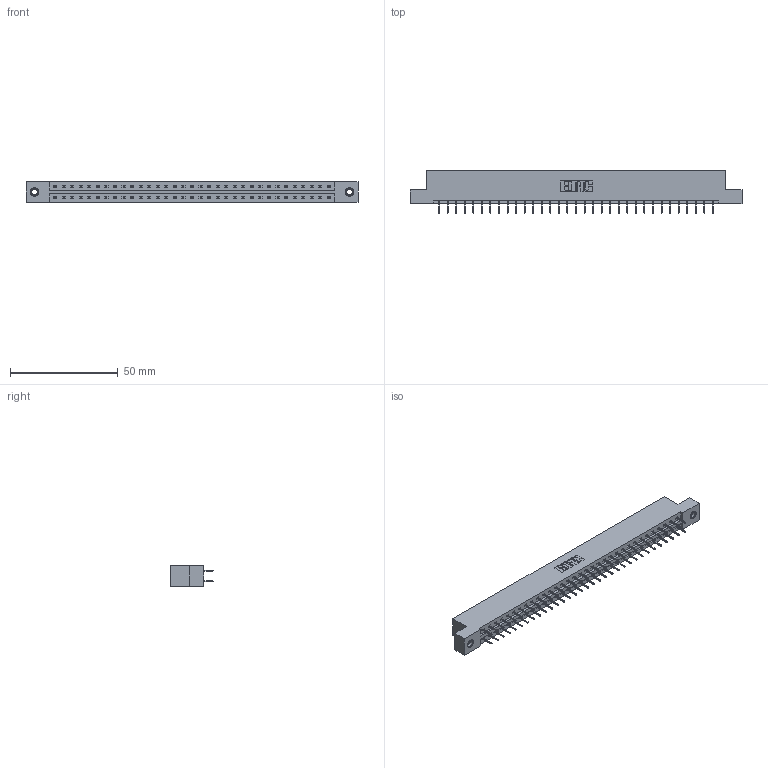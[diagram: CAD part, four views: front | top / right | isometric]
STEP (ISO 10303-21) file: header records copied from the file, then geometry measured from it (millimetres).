
FILE_DESCRIPTION (( 'STEP AP203' ), '1' );
FILE_NAME ('387-066-524-207.STEP', '2019-10-19T18:25:55', ( '' ), ( '' ), 'SwSTEP 2.0', 'SolidWorks 2016', '' );
FILE_SCHEMA (( 'CONFIG_CONTROL_DESIGN' ));
Length unit declared in the file: inch
Products named in the file (4): 345-250-001_345-250-005-103; 345-292-001_345-293-124; 337 Part_Flush Mounting Lugs - 0.156 Dia-TI; 387-066-524-207
Assembly tree (69 placements, depth 2):
  387-066-524-207
    337 Part_Flush Mounting Lugs - 0.156 Dia-TI
    345-292-001_345-293-124  x66
    345-250-001_345-250-005-103  x2
Bounding box: 153.77 x 19.69 x 9.4 mm (x, y, z)
Volume: 15972.5 mm3; surface area: 17696.1 mm2
Topology: 69 solids, 69 shells, 4002 faces, 11337 edges, 7286 vertices
Faces by surface type: plane 3006, cylinder 980, cone 12, torus 4
Entity records: 28010 total; most frequent: CARTESIAN_POINT 4705, ORIENTED_EDGE 4634, DIRECTION 4051, EDGE_CURVE 2317, LINE 2173, VECTOR 2173, VERTEX_POINT 1536, AXIS2_PLACEMENT_3D 939
